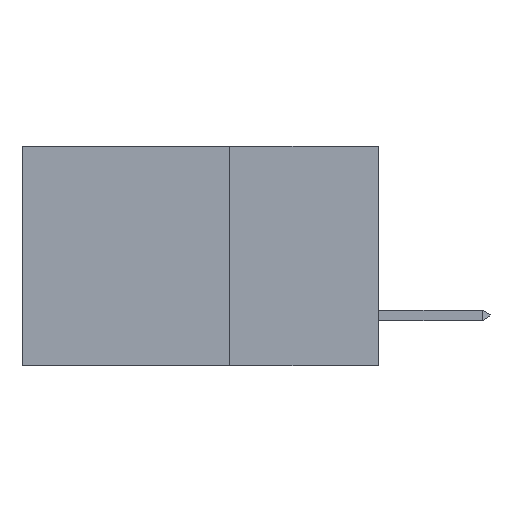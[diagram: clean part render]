
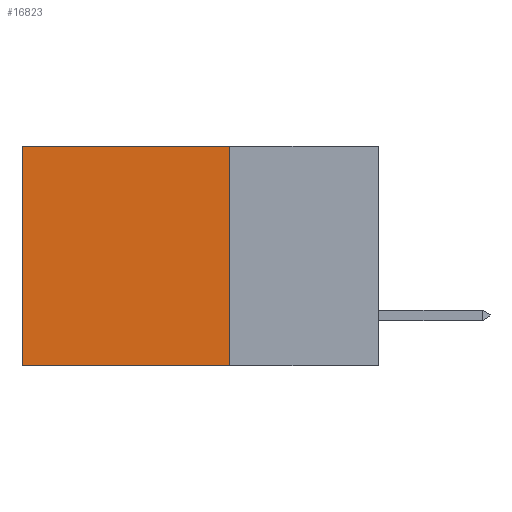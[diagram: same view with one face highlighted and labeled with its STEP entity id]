
A CAD part, left-side view. The second image highlights one B-rep face of the part: STEP entity #16823.
In plain terms, the highlighted planar face has unit normal (-1, 0, 0).
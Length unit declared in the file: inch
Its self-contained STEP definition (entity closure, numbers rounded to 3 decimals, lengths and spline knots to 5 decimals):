
#322 = CARTESIAN_POINT ( 'NONE',  ( 0.298, 0.6, 0. ) ) ;
#468 = DIRECTION ( 'NONE',  ( 1., 0., 0. ) ) ;
#658 = ORIENTED_EDGE ( 'NONE', *, *, #14816, .T. ) ;
#1206 = ORIENTED_EDGE ( 'NONE', *, *, #5571, .T. ) ;
#2645 = FACE_OUTER_BOUND ( 'NONE', #9813, .T. ) ;
#3409 = CARTESIAN_POINT ( 'NONE',  ( 0.298, 0.6, 0. ) ) ;
#3504 = DIRECTION ( 'NONE',  ( 0., 1., 0. ) ) ;
#4177 = VECTOR ( 'NONE', #11610, 39.37008 ) ;
#4362 = LINE ( 'NONE', #322, #9939 ) ;
#4517 = DIRECTION ( 'NONE',  ( 0., 0., -1. ) ) ;
#5450 = LINE ( 'NONE', #15717, #4177 ) ;
#5571 = EDGE_CURVE ( 'NONE', #7481, #9838, #7893, .T. ) ;
#6078 = CARTESIAN_POINT ( 'NONE',  ( 0.298, 0.25, -0.37 ) ) ;
#6329 = CARTESIAN_POINT ( 'NONE',  ( 0.298, 0.25, -0.37 ) ) ;
#6614 = VERTEX_POINT ( 'NONE', #15673 ) ;
#7288 = VECTOR ( 'NONE', #3504, 39.37008 ) ;
#7481 = VERTEX_POINT ( 'NONE', #12146 ) ;
#7893 = LINE ( 'NONE', #15587, #9163 ) ;
#9160 = DIRECTION ( 'NONE',  ( 0., 1., 0. ) ) ;
#9163 = VECTOR ( 'NONE', #9160, 39.37008 ) ;
#9813 = EDGE_LOOP ( 'NONE', ( #658, #15146, #17636, #1206 ) ) ;
#9838 = VERTEX_POINT ( 'NONE', #3409 ) ;
#9939 = VECTOR ( 'NONE', #12454, 39.37008 ) ;
#10455 = EDGE_CURVE ( 'NONE', #14300, #6614, #16329, .T. ) ;
#11204 = AXIS2_PLACEMENT_3D ( 'NONE', #16793, #468, #4517 ) ;
#11610 = DIRECTION ( 'NONE',  ( 0., 0., -1. ) ) ;
#12146 = CARTESIAN_POINT ( 'NONE',  ( 0.298, 0.25, 0. ) ) ;
#12425 = PLANE ( 'NONE',  #11204 ) ;
#12454 = DIRECTION ( 'NONE',  ( 0., 0., -1. ) ) ;
#14124 = EDGE_CURVE ( 'NONE', #7481, #14300, #5450, .T. ) ;
#14300 = VERTEX_POINT ( 'NONE', #6329 ) ;
#14816 = EDGE_CURVE ( 'NONE', #9838, #6614, #4362, .T. ) ;
#15146 = ORIENTED_EDGE ( 'NONE', *, *, #10455, .F. ) ;
#15587 = CARTESIAN_POINT ( 'NONE',  ( 0.298, 0.25, 0. ) ) ;
#15673 = CARTESIAN_POINT ( 'NONE',  ( 0.298, 0.6, -0.37 ) ) ;
#15717 = CARTESIAN_POINT ( 'NONE',  ( 0.298, 0.25, 0. ) ) ;
#16329 = LINE ( 'NONE', #6078, #7288 ) ;
#16793 = CARTESIAN_POINT ( 'NONE',  ( 0.298, 0.25, 0. ) ) ;
#16823 = ADVANCED_FACE ( 'NONE', ( #2645 ), #12425, .F. ) ;
#17636 = ORIENTED_EDGE ( 'NONE', *, *, #14124, .F. ) ;
